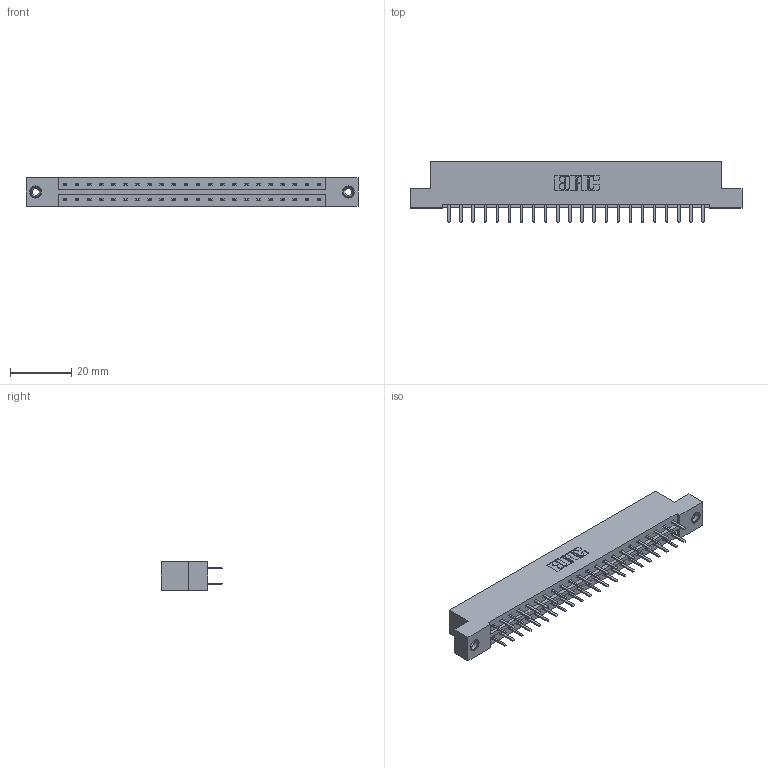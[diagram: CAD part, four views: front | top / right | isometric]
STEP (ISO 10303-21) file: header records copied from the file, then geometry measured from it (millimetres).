
FILE_DESCRIPTION (( 'STEP AP203' ), '1' );
FILE_NAME ('333-044-520-208.STEP', '2018-08-03T20:54:24', ( '' ), ( '' ), 'SwSTEP 2.0', 'SolidWorks 2016', '' );
FILE_SCHEMA (( 'CONFIG_CONTROL_DESIGN' ));
Length unit declared in the file: inch
Products named in the file (4): 333 Part_Flush - .156 Dia - TI; 345-292-001_345-293-120; 345-250-001_345-250-003-102; 333-044-520-208
Assembly tree (47 placements, depth 2):
  333-044-520-208
    333 Part_Flush - .156 Dia - TI
    345-292-001_345-293-120  x44
    345-250-001_345-250-003-102  x2
Bounding box: 108.71 x 20.02 x 9.4 mm (x, y, z)
Volume: 10886 mm3; surface area: 12625.5 mm2
Topology: 47 solids, 47 shells, 2638 faces, 7619 edges, 4954 vertices
Faces by surface type: plane 1774, cylinder 848, cone 12, torus 4
Entity records: 18040 total; most frequent: CARTESIAN_POINT 3009, ORIENTED_EDGE 2926, DIRECTION 2625, EDGE_CURVE 1463, LINE 1311, VECTOR 1311, VERTEX_POINT 968, AXIS2_PLACEMENT_3D 657
